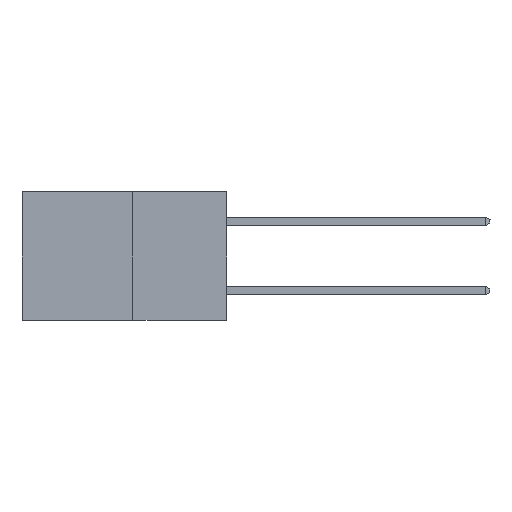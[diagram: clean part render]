
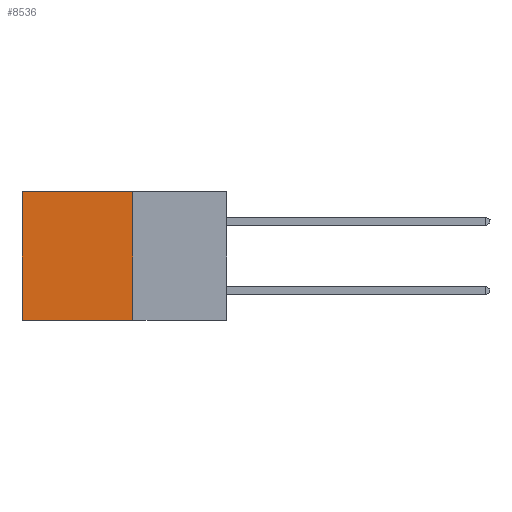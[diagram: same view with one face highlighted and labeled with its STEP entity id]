
A CAD part, left-side view. The second image highlights one B-rep face of the part: STEP entity #8536.
In plain terms, the highlighted planar face has unit normal (-1, 0, 0).
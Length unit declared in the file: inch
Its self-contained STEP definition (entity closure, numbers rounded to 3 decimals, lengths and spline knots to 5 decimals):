
#346 = DIRECTION ( 'NONE',  ( 0., 0., -1. ) ) ;
#1963 = VERTEX_POINT ( 'NONE', #4392 ) ;
#4392 = CARTESIAN_POINT ( 'NONE',  ( 0.277, 0.27, 0. ) ) ;
#5524 = DIRECTION ( 'NONE',  ( 0., 1., 0. ) ) ;
#5614 = DIRECTION ( 'NONE',  ( 0., 0., -1. ) ) ;
#5834 = DIRECTION ( 'NONE',  ( 1., 0., 0. ) ) ;
#5971 = CARTESIAN_POINT ( 'NONE',  ( 0.277, 0.27, -0.37 ) ) ;
#6077 = PLANE ( 'NONE',  #17469 ) ;
#6814 = VECTOR ( 'NONE', #21626, 39.37008 ) ;
#7426 = ORIENTED_EDGE ( 'NONE', *, *, #19183, .F. ) ;
#8198 = LINE ( 'NONE', #10467, #26379 ) ;
#8536 = ADVANCED_FACE ( 'NONE', ( #21428 ), #6077, .F. ) ;
#8632 = CARTESIAN_POINT ( 'NONE',  ( 0.277, 0.27, -0.37 ) ) ;
#9609 = ORIENTED_EDGE ( 'NONE', *, *, #29054, .F. ) ;
#10353 = DIRECTION ( 'NONE',  ( 0., 1., 0. ) ) ;
#10467 = CARTESIAN_POINT ( 'NONE',  ( 0.277, 0.27, -0.37 ) ) ;
#12609 = VERTEX_POINT ( 'NONE', #8632 ) ;
#14228 = LINE ( 'NONE', #16549, #6814 ) ;
#15056 = LINE ( 'NONE', #30298, #15830 ) ;
#15556 = EDGE_CURVE ( 'NONE', #29636, #19973, #14228, .T. ) ;
#15830 = VECTOR ( 'NONE', #346, 39.37008 ) ;
#16549 = CARTESIAN_POINT ( 'NONE',  ( 0.277, 0.59, -0.37 ) ) ;
#17469 = AXIS2_PLACEMENT_3D ( 'NONE', #5971, #5834, #5614 ) ;
#19058 = EDGE_LOOP ( 'NONE', ( #26237, #9609, #7426, #30649 ) ) ;
#19183 = EDGE_CURVE ( 'NONE', #1963, #12609, #15056, .T. ) ;
#19973 = VERTEX_POINT ( 'NONE', #23663 ) ;
#21428 = FACE_OUTER_BOUND ( 'NONE', #19058, .T. ) ;
#21626 = DIRECTION ( 'NONE',  ( 0., 0., -1. ) ) ;
#23663 = CARTESIAN_POINT ( 'NONE',  ( 0.277, 0.59, -0.37 ) ) ;
#24817 = CARTESIAN_POINT ( 'NONE',  ( 0.277, 0.59, 0. ) ) ;
#25405 = EDGE_CURVE ( 'NONE', #1963, #29636, #25696, .T. ) ;
#25696 = LINE ( 'NONE', #30139, #31488 ) ;
#26237 = ORIENTED_EDGE ( 'NONE', *, *, #15556, .T. ) ;
#26379 = VECTOR ( 'NONE', #5524, 39.37008 ) ;
#29054 = EDGE_CURVE ( 'NONE', #12609, #19973, #8198, .T. ) ;
#29636 = VERTEX_POINT ( 'NONE', #24817 ) ;
#30139 = CARTESIAN_POINT ( 'NONE',  ( 0.277, 0.27, 0. ) ) ;
#30298 = CARTESIAN_POINT ( 'NONE',  ( 0.277, 0.27, -0.37 ) ) ;
#30649 = ORIENTED_EDGE ( 'NONE', *, *, #25405, .T. ) ;
#31488 = VECTOR ( 'NONE', #10353, 39.37008 ) ;
